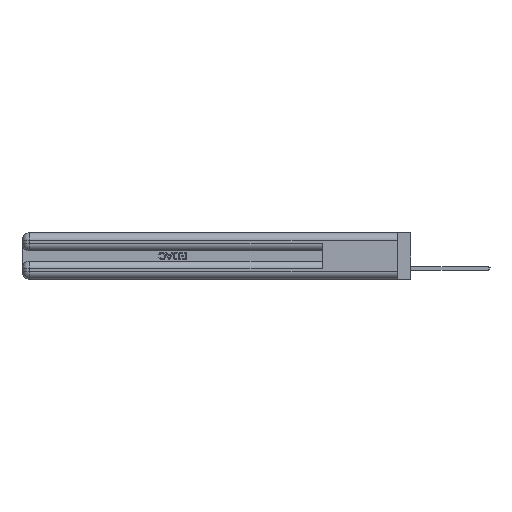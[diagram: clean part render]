
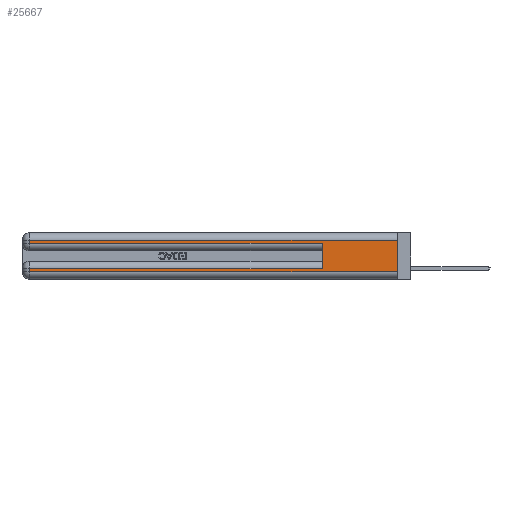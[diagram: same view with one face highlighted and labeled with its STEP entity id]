
A CAD part, left-side view. The second image highlights one B-rep face of the part: STEP entity #25667.
In plain terms, the highlighted planar face has unit normal (-1, 0, 0).
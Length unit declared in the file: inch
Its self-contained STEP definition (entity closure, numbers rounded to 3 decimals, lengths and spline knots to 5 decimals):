
#730 = FACE_OUTER_BOUND ( 'NONE', #44416, .T. ) ;
#2021 = CARTESIAN_POINT ( 'NONE',  ( 0., 2.94, 0.085 ) ) ;
#3722 = EDGE_CURVE ( 'NONE', #40703, #12180, #7223, .T. ) ;
#3884 = ORIENTED_EDGE ( 'NONE', *, *, #3722, .F. ) ;
#4754 = AXIS2_PLACEMENT_3D ( 'NONE', #13323, #38203, #44916 ) ;
#5391 = DIRECTION ( 'NONE',  ( 0., 0., -1. ) ) ;
#5438 = CARTESIAN_POINT ( 'NONE',  ( 0., 0., 0.06 ) ) ;
#5446 = LINE ( 'NONE', #39729, #43448 ) ;
#5532 = EDGE_CURVE ( 'NONE', #34415, #27787, #5446, .T. ) ;
#5837 = VECTOR ( 'NONE', #23402, 39.37008 ) ;
#5894 = DIRECTION ( 'NONE',  ( 0., 0., 1. ) ) ;
#6257 = LINE ( 'NONE', #38917, #25818 ) ;
#6442 = CARTESIAN_POINT ( 'NONE',  ( 0., 2.94, 0.37 ) ) ;
#6708 = ORIENTED_EDGE ( 'NONE', *, *, #5532, .T. ) ;
#7223 = LINE ( 'NONE', #43956, #11580 ) ;
#8315 = EDGE_CURVE ( 'NONE', #27787, #38641, #6257, .T. ) ;
#9074 = CARTESIAN_POINT ( 'NONE',  ( 0., 2.94, 0.31 ) ) ;
#9411 = ORIENTED_EDGE ( 'NONE', *, *, #16268, .T. ) ;
#10458 = VECTOR ( 'NONE', #29422, 39.37008 ) ;
#11309 = VERTEX_POINT ( 'NONE', #33933 ) ;
#11580 = VECTOR ( 'NONE', #5894, 39.37008 ) ;
#12180 = VERTEX_POINT ( 'NONE', #14671 ) ;
#12283 = EDGE_CURVE ( 'NONE', #11309, #38641, #28915, .T. ) ;
#12626 = DIRECTION ( 'NONE',  ( 0., 1., 0. ) ) ;
#13323 = CARTESIAN_POINT ( 'NONE',  ( 0., 0., 0.37 ) ) ;
#13514 = ORIENTED_EDGE ( 'NONE', *, *, #20426, .T. ) ;
#14671 = CARTESIAN_POINT ( 'NONE',  ( 0., 0.6, 0.285 ) ) ;
#14947 = LINE ( 'NONE', #6442, #5837 ) ;
#15718 = ORIENTED_EDGE ( 'NONE', *, *, #35932, .T. ) ;
#16268 = EDGE_CURVE ( 'NONE', #43510, #12180, #42472, .T. ) ;
#16436 = VECTOR ( 'NONE', #41251, 39.37008 ) ;
#20426 = EDGE_CURVE ( 'NONE', #20680, #43510, #14947, .T. ) ;
#20680 = VERTEX_POINT ( 'NONE', #9074 ) ;
#21121 = CARTESIAN_POINT ( 'NONE',  ( 0., 0., 0.285 ) ) ;
#21761 = PLANE ( 'NONE',  #4754 ) ;
#21895 = ORIENTED_EDGE ( 'NONE', *, *, #23004, .T. ) ;
#23004 = EDGE_CURVE ( 'NONE', #11309, #20680, #39634, .T. ) ;
#23132 = CARTESIAN_POINT ( 'NONE',  ( 0., 2.94, 0.06 ) ) ;
#23402 = DIRECTION ( 'NONE',  ( 0., 0., -1. ) ) ;
#25025 = CARTESIAN_POINT ( 'NONE',  ( 0., 2.94, 0.285 ) ) ;
#25667 = ADVANCED_FACE ( 'NONE', ( #730 ), #21761, .F. ) ;
#25818 = VECTOR ( 'NONE', #42362, 39.37008 ) ;
#27078 = CARTESIAN_POINT ( 'NONE',  ( 0., 0., 0.085 ) ) ;
#27787 = VERTEX_POINT ( 'NONE', #23132 ) ;
#28915 = LINE ( 'NONE', #30034, #10458 ) ;
#29422 = DIRECTION ( 'NONE',  ( 0., 0., -1. ) ) ;
#30034 = CARTESIAN_POINT ( 'NONE',  ( 0., 0., 0.37 ) ) ;
#33274 = DIRECTION ( 'NONE',  ( 0., 1., 0. ) ) ;
#33933 = CARTESIAN_POINT ( 'NONE',  ( 0., 0., 0.31 ) ) ;
#34415 = VERTEX_POINT ( 'NONE', #2021 ) ;
#34837 = VECTOR ( 'NONE', #33274, 39.37008 ) ;
#35932 = EDGE_CURVE ( 'NONE', #40703, #34415, #37030, .T. ) ;
#36984 = CARTESIAN_POINT ( 'NONE',  ( 0., 0., 0.31 ) ) ;
#37030 = LINE ( 'NONE', #27078, #34837 ) ;
#37343 = CARTESIAN_POINT ( 'NONE',  ( 0., 0.6, 0.085 ) ) ;
#38203 = DIRECTION ( 'NONE',  ( 1., 0., 0. ) ) ;
#38641 = VERTEX_POINT ( 'NONE', #5438 ) ;
#38917 = CARTESIAN_POINT ( 'NONE',  ( 0., 0., 0.06 ) ) ;
#39091 = VECTOR ( 'NONE', #12626, 39.37008 ) ;
#39287 = ORIENTED_EDGE ( 'NONE', *, *, #12283, .F. ) ;
#39634 = LINE ( 'NONE', #36984, #39091 ) ;
#39729 = CARTESIAN_POINT ( 'NONE',  ( 0., 2.94, 0.37 ) ) ;
#40703 = VERTEX_POINT ( 'NONE', #37343 ) ;
#41251 = DIRECTION ( 'NONE',  ( 0., -1., 0. ) ) ;
#41977 = ORIENTED_EDGE ( 'NONE', *, *, #8315, .T. ) ;
#42362 = DIRECTION ( 'NONE',  ( 0., -1., 0. ) ) ;
#42472 = LINE ( 'NONE', #21121, #16436 ) ;
#43448 = VECTOR ( 'NONE', #5391, 39.37008 ) ;
#43510 = VERTEX_POINT ( 'NONE', #25025 ) ;
#43956 = CARTESIAN_POINT ( 'NONE',  ( 0., 0.6, 0.145 ) ) ;
#44416 = EDGE_LOOP ( 'NONE', ( #39287, #21895, #13514, #9411, #3884, #15718, #6708, #41977 ) ) ;
#44916 = DIRECTION ( 'NONE',  ( 0., 0., -1. ) ) ;
